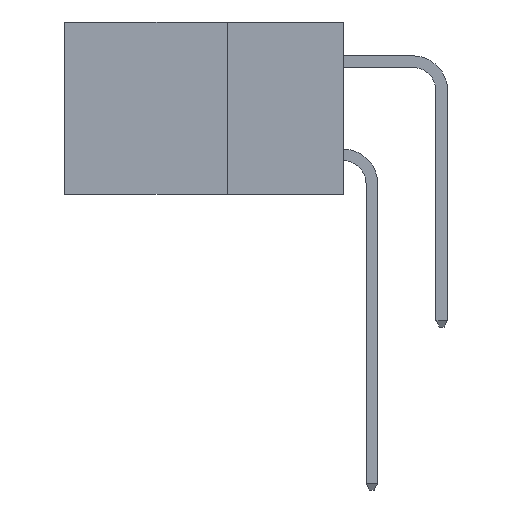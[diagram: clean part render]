
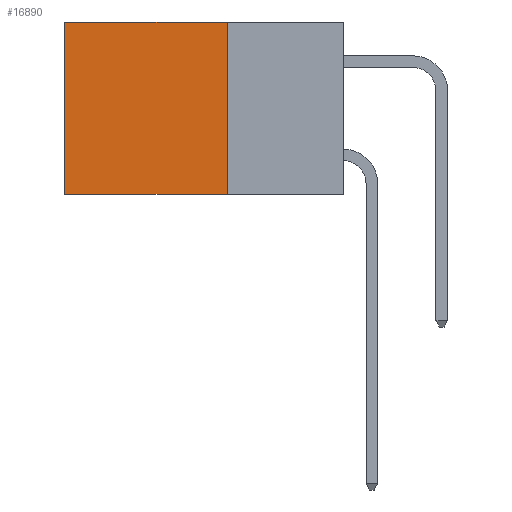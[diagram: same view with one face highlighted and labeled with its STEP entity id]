
A CAD part, left-side view. The second image highlights one B-rep face of the part: STEP entity #16890.
In plain terms, the highlighted planar face has unit normal (-1, 0, 0).
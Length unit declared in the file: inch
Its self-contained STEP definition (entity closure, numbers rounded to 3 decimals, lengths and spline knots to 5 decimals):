
#890 = VECTOR ( 'NONE', #17926, 39.37008 ) ;
#2317 = EDGE_LOOP ( 'NONE', ( #17161, #18450, #5235, #5466 ) ) ;
#3197 = CARTESIAN_POINT ( 'NONE',  ( 0.2615, 0.25, -0.37 ) ) ;
#3486 = CARTESIAN_POINT ( 'NONE',  ( 0.2615, 0.25, -0.37 ) ) ;
#3487 = LINE ( 'NONE', #4595, #15833 ) ;
#4595 = CARTESIAN_POINT ( 'NONE',  ( 0.2615, 0.25, -0.37 ) ) ;
#4827 = LINE ( 'NONE', #11750, #17100 ) ;
#5219 = DIRECTION ( 'NONE',  ( 0., 0., -1. ) ) ;
#5235 = ORIENTED_EDGE ( 'NONE', *, *, #6703, .F. ) ;
#5398 = VECTOR ( 'NONE', #19367, 39.37008 ) ;
#5466 = ORIENTED_EDGE ( 'NONE', *, *, #14248, .T. ) ;
#6530 = EDGE_CURVE ( 'NONE', #7629, #13660, #3487, .T. ) ;
#6703 = EDGE_CURVE ( 'NONE', #19330, #7629, #4827, .T. ) ;
#7629 = VERTEX_POINT ( 'NONE', #3197 ) ;
#7907 = CARTESIAN_POINT ( 'NONE',  ( 0.2615, 0.6, -0.37 ) ) ;
#8449 = CARTESIAN_POINT ( 'NONE',  ( 0.2615, 0.6, 0. ) ) ;
#8611 = AXIS2_PLACEMENT_3D ( 'NONE', #3486, #15237, #5219 ) ;
#11750 = CARTESIAN_POINT ( 'NONE',  ( 0.2615, 0.25, -0.37 ) ) ;
#13417 = DIRECTION ( 'NONE',  ( 0., 0., -1. ) ) ;
#13581 = PLANE ( 'NONE',  #8611 ) ;
#13660 = VERTEX_POINT ( 'NONE', #19709 ) ;
#14248 = EDGE_CURVE ( 'NONE', #19330, #18753, #14371, .T. ) ;
#14371 = LINE ( 'NONE', #16296, #890 ) ;
#14817 = LINE ( 'NONE', #7907, #5398 ) ;
#15222 = CARTESIAN_POINT ( 'NONE',  ( 0.2615, 0.25, 0. ) ) ;
#15237 = DIRECTION ( 'NONE',  ( 1., 0., 0. ) ) ;
#15276 = FACE_OUTER_BOUND ( 'NONE', #2317, .T. ) ;
#15597 = EDGE_CURVE ( 'NONE', #18753, #13660, #14817, .T. ) ;
#15833 = VECTOR ( 'NONE', #19577, 39.37008 ) ;
#16296 = CARTESIAN_POINT ( 'NONE',  ( 0.2615, 0.25, 0. ) ) ;
#16890 = ADVANCED_FACE ( 'NONE', ( #15276 ), #13581, .F. ) ;
#17100 = VECTOR ( 'NONE', #13417, 39.37008 ) ;
#17161 = ORIENTED_EDGE ( 'NONE', *, *, #15597, .T. ) ;
#17926 = DIRECTION ( 'NONE',  ( 0., 1., 0. ) ) ;
#18450 = ORIENTED_EDGE ( 'NONE', *, *, #6530, .F. ) ;
#18753 = VERTEX_POINT ( 'NONE', #8449 ) ;
#19330 = VERTEX_POINT ( 'NONE', #15222 ) ;
#19367 = DIRECTION ( 'NONE',  ( 0., 0., -1. ) ) ;
#19577 = DIRECTION ( 'NONE',  ( 0., 1., 0. ) ) ;
#19709 = CARTESIAN_POINT ( 'NONE',  ( 0.2615, 0.6, -0.37 ) ) ;
